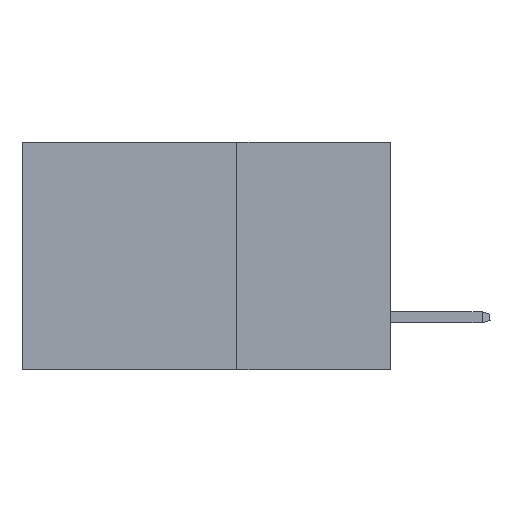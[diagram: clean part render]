
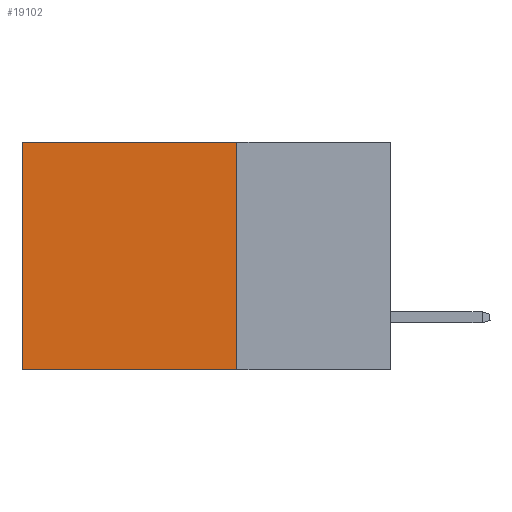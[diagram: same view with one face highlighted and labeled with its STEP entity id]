
A CAD part, left-side view. The second image highlights one B-rep face of the part: STEP entity #19102.
In plain terms, the highlighted planar face has unit normal (-1, 0, 0).
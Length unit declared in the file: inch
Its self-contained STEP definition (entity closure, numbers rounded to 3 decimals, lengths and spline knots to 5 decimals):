
#1215 = ORIENTED_EDGE ( 'NONE', *, *, #16412, .F. ) ;
#1847 = DIRECTION ( 'NONE',  ( 1., 0., 0. ) ) ;
#3469 = VECTOR ( 'NONE', #5933, 39.37008 ) ;
#4155 = CARTESIAN_POINT ( 'NONE',  ( 0.2875, 0.6, 0. ) ) ;
#4459 = LINE ( 'NONE', #16022, #8451 ) ;
#5398 = EDGE_CURVE ( 'NONE', #19997, #17906, #14196, .T. ) ;
#5933 = DIRECTION ( 'NONE',  ( 0., 0., -1. ) ) ;
#6703 = VECTOR ( 'NONE', #14615, 39.37008 ) ;
#7517 = EDGE_CURVE ( 'NONE', #21676, #19997, #4459, .T. ) ;
#8451 = VECTOR ( 'NONE', #23010, 39.37008 ) ;
#9479 = LINE ( 'NONE', #20029, #6703 ) ;
#9564 = CARTESIAN_POINT ( 'NONE',  ( 0.2875, 0.25, 0. ) ) ;
#10163 = ORIENTED_EDGE ( 'NONE', *, *, #21974, .F. ) ;
#10686 = PLANE ( 'NONE',  #16925 ) ;
#11181 = ORIENTED_EDGE ( 'NONE', *, *, #5398, .T. ) ;
#11277 = LINE ( 'NONE', #16511, #3469 ) ;
#14196 = LINE ( 'NONE', #18384, #22516 ) ;
#14615 = DIRECTION ( 'NONE',  ( 0., 1., 0. ) ) ;
#15364 = DIRECTION ( 'NONE',  ( 0., 0., -1. ) ) ;
#15618 = DIRECTION ( 'NONE',  ( 0., 0., -1. ) ) ;
#16022 = CARTESIAN_POINT ( 'NONE',  ( 0.2875, 0.25, 0. ) ) ;
#16362 = VERTEX_POINT ( 'NONE', #20903 ) ;
#16412 = EDGE_CURVE ( 'NONE', #16362, #17906, #9479, .T. ) ;
#16511 = CARTESIAN_POINT ( 'NONE',  ( 0.2875, 0.25, 0. ) ) ;
#16599 = FACE_OUTER_BOUND ( 'NONE', #19348, .T. ) ;
#16925 = AXIS2_PLACEMENT_3D ( 'NONE', #17798, #1847, #15364 ) ;
#17798 = CARTESIAN_POINT ( 'NONE',  ( 0.2875, 0.25, 0. ) ) ;
#17906 = VERTEX_POINT ( 'NONE', #20020 ) ;
#18384 = CARTESIAN_POINT ( 'NONE',  ( 0.2875, 0.6, 0. ) ) ;
#19102 = ADVANCED_FACE ( 'NONE', ( #16599 ), #10686, .F. ) ;
#19348 = EDGE_LOOP ( 'NONE', ( #11181, #1215, #10163, #20888 ) ) ;
#19997 = VERTEX_POINT ( 'NONE', #4155 ) ;
#20020 = CARTESIAN_POINT ( 'NONE',  ( 0.2875, 0.6, -0.37 ) ) ;
#20029 = CARTESIAN_POINT ( 'NONE',  ( 0.2875, 0.25, -0.37 ) ) ;
#20888 = ORIENTED_EDGE ( 'NONE', *, *, #7517, .T. ) ;
#20903 = CARTESIAN_POINT ( 'NONE',  ( 0.2875, 0.25, -0.37 ) ) ;
#21676 = VERTEX_POINT ( 'NONE', #9564 ) ;
#21974 = EDGE_CURVE ( 'NONE', #21676, #16362, #11277, .T. ) ;
#22516 = VECTOR ( 'NONE', #15618, 39.37008 ) ;
#23010 = DIRECTION ( 'NONE',  ( 0., 1., 0. ) ) ;
